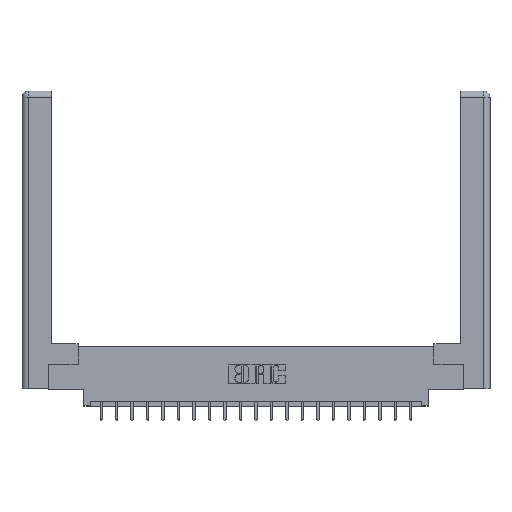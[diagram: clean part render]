
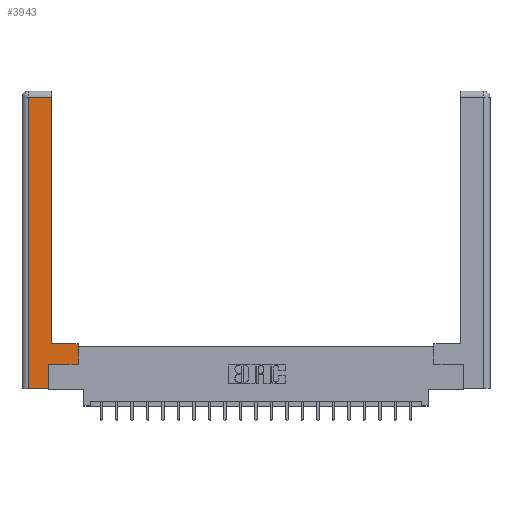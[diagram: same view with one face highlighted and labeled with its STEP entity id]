
A CAD part, top view. The second image highlights one B-rep face of the part: STEP entity #3943.
In plain terms, the highlighted planar face has unit normal (0, 0, 1).
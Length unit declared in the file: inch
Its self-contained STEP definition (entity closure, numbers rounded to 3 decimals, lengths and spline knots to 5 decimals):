
#536 = EDGE_CURVE ( 'NONE', #2082, #12078, #2633, .T. ) ;
#1000 = DIRECTION ( 'NONE',  ( 1., 0., 0. ) ) ;
#1843 = DIRECTION ( 'NONE',  ( -1., 0., 0. ) ) ;
#1867 = PLANE ( 'NONE',  #3105 ) ;
#1871 = ORIENTED_EDGE ( 'NONE', *, *, #19362, .T. ) ;
#2047 = VERTEX_POINT ( 'NONE', #14600 ) ;
#2082 = VERTEX_POINT ( 'NONE', #13343 ) ;
#2633 = LINE ( 'NONE', #9699, #11040 ) ;
#2640 = CARTESIAN_POINT ( 'NONE',  ( 0.265, 0.245, 0. ) ) ;
#2895 = CARTESIAN_POINT ( 'NONE',  ( 0.265, 0., 0. ) ) ;
#2976 = VECTOR ( 'NONE', #4631, 39.37008 ) ;
#3049 = ORIENTED_EDGE ( 'NONE', *, *, #7199, .T. ) ;
#3051 = LINE ( 'NONE', #3262, #13269 ) ;
#3105 = AXIS2_PLACEMENT_3D ( 'NONE', #18686, #11865, #5392 ) ;
#3180 = DIRECTION ( 'NONE',  ( 0., 1., 0. ) ) ;
#3262 = CARTESIAN_POINT ( 'NONE',  ( 0.295, 3., 0. ) ) ;
#3719 = ORIENTED_EDGE ( 'NONE', *, *, #21704, .T. ) ;
#3856 = ORIENTED_EDGE ( 'NONE', *, *, #12630, .T. ) ;
#3943 = ADVANCED_FACE ( 'NONE', ( #6592 ), #1867, .F. ) ;
#4102 = ORIENTED_EDGE ( 'NONE', *, *, #17621, .T. ) ;
#4631 = DIRECTION ( 'NONE',  ( 1., 0., 0. ) ) ;
#4794 = EDGE_CURVE ( 'NONE', #9827, #2047, #7998, .T. ) ;
#5046 = CARTESIAN_POINT ( 'NONE',  ( 0.0615, 0., 0. ) ) ;
#5392 = DIRECTION ( 'NONE',  ( -1., 0., 0. ) ) ;
#6592 = FACE_OUTER_BOUND ( 'NONE', #11951, .T. ) ;
#6696 = CARTESIAN_POINT ( 'NONE',  ( 0.295, 0.45, 0. ) ) ;
#7199 = EDGE_CURVE ( 'NONE', #9690, #2082, #13396, .T. ) ;
#7998 = LINE ( 'NONE', #2895, #2976 ) ;
#8977 = ORIENTED_EDGE ( 'NONE', *, *, #536, .T. ) ;
#9690 = VERTEX_POINT ( 'NONE', #17378 ) ;
#9699 = CARTESIAN_POINT ( 'NONE',  ( 0.295, 0.45, 0. ) ) ;
#9827 = VERTEX_POINT ( 'NONE', #15037 ) ;
#10647 = CARTESIAN_POINT ( 'NONE',  ( 0.295, 2.94, 0. ) ) ;
#10839 = VECTOR ( 'NONE', #1843, 39.37008 ) ;
#11040 = VECTOR ( 'NONE', #14727, 39.37008 ) ;
#11377 = LINE ( 'NONE', #16970, #10839 ) ;
#11505 = VERTEX_POINT ( 'NONE', #10647 ) ;
#11865 = DIRECTION ( 'NONE',  ( 0., 0., -1. ) ) ;
#11951 = EDGE_LOOP ( 'NONE', ( #1871, #3719, #15980, #17201, #3856, #4102, #3049, #8977 ) ) ;
#12078 = VERTEX_POINT ( 'NONE', #6696 ) ;
#12630 = EDGE_CURVE ( 'NONE', #2047, #19907, #21210, .T. ) ;
#12908 = CARTESIAN_POINT ( 'NONE',  ( 0.0615, 2.94, 0. ) ) ;
#13269 = VECTOR ( 'NONE', #3180, 39.37008 ) ;
#13343 = CARTESIAN_POINT ( 'NONE',  ( 0.565, 0.45, 0. ) ) ;
#13396 = LINE ( 'NONE', #15065, #15496 ) ;
#13827 = VECTOR ( 'NONE', #21011, 39.37008 ) ;
#14250 = VERTEX_POINT ( 'NONE', #12908 ) ;
#14408 = EDGE_CURVE ( 'NONE', #14250, #9827, #18469, .T. ) ;
#14600 = CARTESIAN_POINT ( 'NONE',  ( 0.265, 0., 0. ) ) ;
#14654 = VECTOR ( 'NONE', #1000, 39.37008 ) ;
#14727 = DIRECTION ( 'NONE',  ( -1., 0., 0. ) ) ;
#14848 = DIRECTION ( 'NONE',  ( 0., 1., 0. ) ) ;
#15037 = CARTESIAN_POINT ( 'NONE',  ( 0.0615, 0., 0. ) ) ;
#15065 = CARTESIAN_POINT ( 'NONE',  ( 0.565, 0.45, 0. ) ) ;
#15293 = VECTOR ( 'NONE', #21711, 39.37008 ) ;
#15496 = VECTOR ( 'NONE', #14848, 39.37008 ) ;
#15968 = CARTESIAN_POINT ( 'NONE',  ( 0.265, 0.245, 0. ) ) ;
#15980 = ORIENTED_EDGE ( 'NONE', *, *, #14408, .T. ) ;
#16970 = CARTESIAN_POINT ( 'NONE',  ( 0.0615, 2.94, 0. ) ) ;
#17201 = ORIENTED_EDGE ( 'NONE', *, *, #4794, .T. ) ;
#17378 = CARTESIAN_POINT ( 'NONE',  ( 0.565, 0.245, 0. ) ) ;
#17621 = EDGE_CURVE ( 'NONE', #19907, #9690, #20184, .T. ) ;
#17738 = CARTESIAN_POINT ( 'NONE',  ( 0.565, 0.245, 0. ) ) ;
#18469 = LINE ( 'NONE', #5046, #15293 ) ;
#18686 = CARTESIAN_POINT ( 'NONE',  ( 0., 0., 0. ) ) ;
#19362 = EDGE_CURVE ( 'NONE', #12078, #11505, #3051, .T. ) ;
#19907 = VERTEX_POINT ( 'NONE', #15968 ) ;
#20184 = LINE ( 'NONE', #17738, #14654 ) ;
#21011 = DIRECTION ( 'NONE',  ( 0., 1., 0. ) ) ;
#21210 = LINE ( 'NONE', #2640, #13827 ) ;
#21704 = EDGE_CURVE ( 'NONE', #11505, #14250, #11377, .T. ) ;
#21711 = DIRECTION ( 'NONE',  ( 0., -1., 0. ) ) ;
